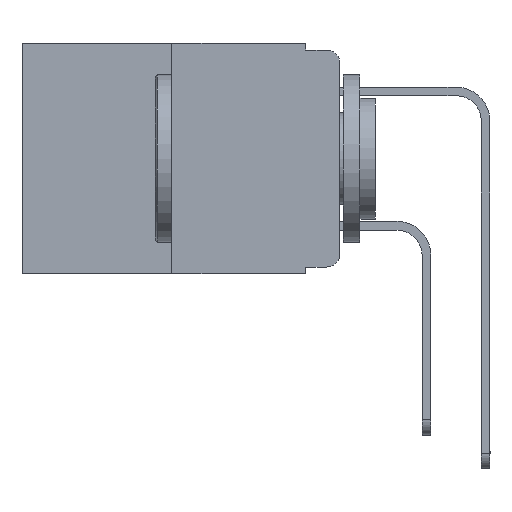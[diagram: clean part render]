
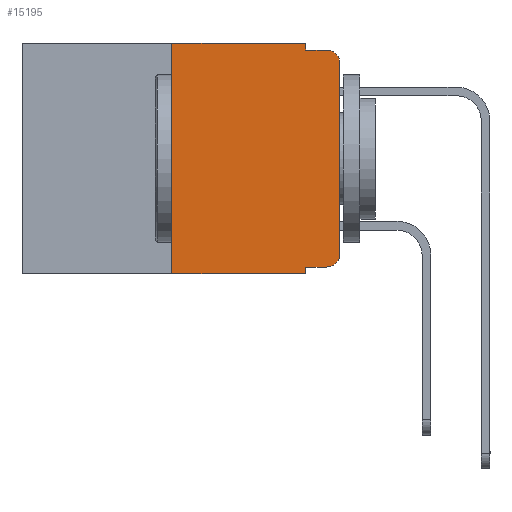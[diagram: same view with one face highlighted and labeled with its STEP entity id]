
A CAD part, left-side view. The second image highlights one B-rep face of the part: STEP entity #15195.
In plain terms, the highlighted planar face has unit normal (-1, 0, 0).
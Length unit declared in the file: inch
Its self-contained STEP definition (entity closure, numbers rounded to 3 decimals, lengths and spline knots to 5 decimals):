
#322 = VERTEX_POINT ( 'NONE', #2821 ) ;
#357 = VECTOR ( 'NONE', #10622, 39.37008 ) ;
#618 = VERTEX_POINT ( 'NONE', #10405 ) ;
#708 = DIRECTION ( 'NONE',  ( 0., 0., 1. ) ) ;
#936 = CARTESIAN_POINT ( 'NONE',  ( 0., 0.473, 0. ) ) ;
#1756 = DIRECTION ( 'NONE',  ( 1., 0., 0. ) ) ;
#1850 = AXIS2_PLACEMENT_3D ( 'NONE', #5429, #13435, #19993 ) ;
#2263 = VECTOR ( 'NONE', #18653, 39.37008 ) ;
#2502 = LINE ( 'NONE', #9144, #4041 ) ;
#2821 = CARTESIAN_POINT ( 'NONE',  ( 0., 0.25, 0. ) ) ;
#3122 = DIRECTION ( 'NONE',  ( 0., 0., -1. ) ) ;
#3392 = DIRECTION ( 'NONE',  ( 0., -1., 0. ) ) ;
#3453 = LINE ( 'NONE', #15181, #12575 ) ;
#3815 = EDGE_LOOP ( 'NONE', ( #11724, #5077, #11843, #13011, #20528, #10294, #8457, #8525, #9364, #21285 ) ) ;
#3984 = VERTEX_POINT ( 'NONE', #12108 ) ;
#4041 = VECTOR ( 'NONE', #5996, 39.37008 ) ;
#4767 = LINE ( 'NONE', #11389, #9837 ) ;
#5077 = ORIENTED_EDGE ( 'NONE', *, *, #8945, .T. ) ;
#5137 = VERTEX_POINT ( 'NONE', #10383 ) ;
#5347 = CARTESIAN_POINT ( 'NONE',  ( 0., 0.02, -0.333 ) ) ;
#5429 = CARTESIAN_POINT ( 'NONE',  ( 0., 0.02, -0.03 ) ) ;
#5996 = DIRECTION ( 'NONE',  ( 0., 0., 1. ) ) ;
#6984 = EDGE_CURVE ( 'NONE', #12755, #618, #19959, .T. ) ;
#7453 = CARTESIAN_POINT ( 'NONE',  ( 0., 0.25, -0.343 ) ) ;
#8206 = CARTESIAN_POINT ( 'NONE',  ( 0., 0.473, -0.343 ) ) ;
#8271 = AXIS2_PLACEMENT_3D ( 'NONE', #12632, #14481, #15879 ) ;
#8457 = ORIENTED_EDGE ( 'NONE', *, *, #16662, .T. ) ;
#8525 = ORIENTED_EDGE ( 'NONE', *, *, #8932, .F. ) ;
#8656 = CARTESIAN_POINT ( 'NONE',  ( 0., 0.051, -0.01 ) ) ;
#8875 = CARTESIAN_POINT ( 'NONE',  ( 0., 0.25, 0. ) ) ;
#8932 = EDGE_CURVE ( 'NONE', #19486, #3984, #4767, .T. ) ;
#8938 = CIRCLE ( 'NONE', #8271, 0.02 ) ;
#8945 = EDGE_CURVE ( 'NONE', #20013, #618, #10511, .T. ) ;
#8997 = LINE ( 'NONE', #20844, #12235 ) ;
#9144 = CARTESIAN_POINT ( 'NONE',  ( 0., 0., 0. ) ) ;
#9364 = ORIENTED_EDGE ( 'NONE', *, *, #10324, .T. ) ;
#9592 = DIRECTION ( 'NONE',  ( 0., 0., -1. ) ) ;
#9805 = PLANE ( 'NONE',  #15167 ) ;
#9837 = VECTOR ( 'NONE', #3122, 39.37008 ) ;
#10294 = ORIENTED_EDGE ( 'NONE', *, *, #13121, .F. ) ;
#10324 = EDGE_CURVE ( 'NONE', #19486, #19152, #3453, .T. ) ;
#10383 = CARTESIAN_POINT ( 'NONE',  ( 0., 0., -0.313 ) ) ;
#10405 = CARTESIAN_POINT ( 'NONE',  ( 0., 0.02, -0.01 ) ) ;
#10511 = CIRCLE ( 'NONE', #1850, 0.02 ) ;
#10539 = EDGE_CURVE ( 'NONE', #15512, #12755, #8997, .T. ) ;
#10622 = DIRECTION ( 'NONE',  ( 0., -1., 0. ) ) ;
#11285 = CARTESIAN_POINT ( 'NONE',  ( 0., 0.051, -0.333 ) ) ;
#11389 = CARTESIAN_POINT ( 'NONE',  ( 0., 0.051, 0. ) ) ;
#11724 = ORIENTED_EDGE ( 'NONE', *, *, #14186, .T. ) ;
#11843 = ORIENTED_EDGE ( 'NONE', *, *, #6984, .F. ) ;
#12108 = CARTESIAN_POINT ( 'NONE',  ( 0., 0.051, -0.343 ) ) ;
#12235 = VECTOR ( 'NONE', #13879, 39.37008 ) ;
#12575 = VECTOR ( 'NONE', #15383, 39.37008 ) ;
#12632 = CARTESIAN_POINT ( 'NONE',  ( 0., 0.02, -0.313 ) ) ;
#12755 = VERTEX_POINT ( 'NONE', #13578 ) ;
#13011 = ORIENTED_EDGE ( 'NONE', *, *, #10539, .F. ) ;
#13025 = VECTOR ( 'NONE', #708, 39.37008 ) ;
#13121 = EDGE_CURVE ( 'NONE', #16261, #322, #17237, .T. ) ;
#13435 = DIRECTION ( 'NONE',  ( -1., 0., 0. ) ) ;
#13527 = CARTESIAN_POINT ( 'NONE',  ( 0., 0., -0.03 ) ) ;
#13578 = CARTESIAN_POINT ( 'NONE',  ( 0., 0.051, -0.01 ) ) ;
#13879 = DIRECTION ( 'NONE',  ( 0., 0., -1. ) ) ;
#14186 = EDGE_CURVE ( 'NONE', #5137, #20013, #2502, .T. ) ;
#14481 = DIRECTION ( 'NONE',  ( -1., 0., 0. ) ) ;
#15167 = AXIS2_PLACEMENT_3D ( 'NONE', #17973, #1756, #9592 ) ;
#15181 = CARTESIAN_POINT ( 'NONE',  ( 0., 0.051, -0.333 ) ) ;
#15195 = ADVANCED_FACE ( 'NONE', ( #21450 ), #9805, .F. ) ;
#15383 = DIRECTION ( 'NONE',  ( 0., -1., 0. ) ) ;
#15512 = VERTEX_POINT ( 'NONE', #19382 ) ;
#15879 = DIRECTION ( 'NONE',  ( 0., 0., -1. ) ) ;
#16261 = VERTEX_POINT ( 'NONE', #7453 ) ;
#16372 = EDGE_CURVE ( 'NONE', #19152, #5137, #8938, .T. ) ;
#16431 = LINE ( 'NONE', #8206, #16576 ) ;
#16576 = VECTOR ( 'NONE', #3392, 39.37008 ) ;
#16662 = EDGE_CURVE ( 'NONE', #16261, #3984, #16431, .T. ) ;
#17237 = LINE ( 'NONE', #8875, #13025 ) ;
#17687 = LINE ( 'NONE', #936, #357 ) ;
#17973 = CARTESIAN_POINT ( 'NONE',  ( 0., 0.473, 0. ) ) ;
#18653 = DIRECTION ( 'NONE',  ( 0., -1., 0. ) ) ;
#19152 = VERTEX_POINT ( 'NONE', #5347 ) ;
#19382 = CARTESIAN_POINT ( 'NONE',  ( 0., 0.051, 0. ) ) ;
#19486 = VERTEX_POINT ( 'NONE', #11285 ) ;
#19659 = EDGE_CURVE ( 'NONE', #322, #15512, #17687, .T. ) ;
#19959 = LINE ( 'NONE', #8656, #2263 ) ;
#19993 = DIRECTION ( 'NONE',  ( 0., 0., -1. ) ) ;
#20013 = VERTEX_POINT ( 'NONE', #13527 ) ;
#20528 = ORIENTED_EDGE ( 'NONE', *, *, #19659, .F. ) ;
#20844 = CARTESIAN_POINT ( 'NONE',  ( 0., 0.051, 0. ) ) ;
#21285 = ORIENTED_EDGE ( 'NONE', *, *, #16372, .T. ) ;
#21450 = FACE_OUTER_BOUND ( 'NONE', #3815, .T. ) ;
